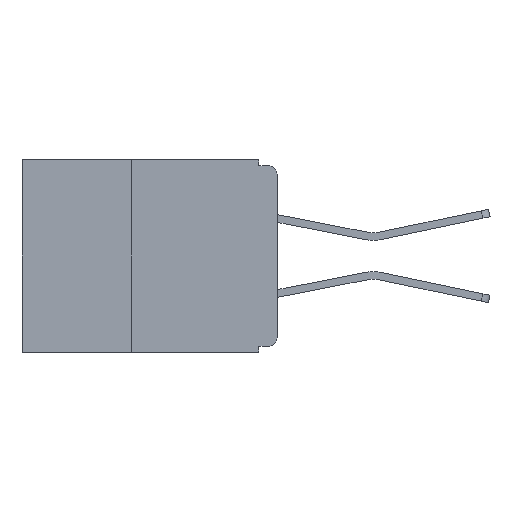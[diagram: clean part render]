
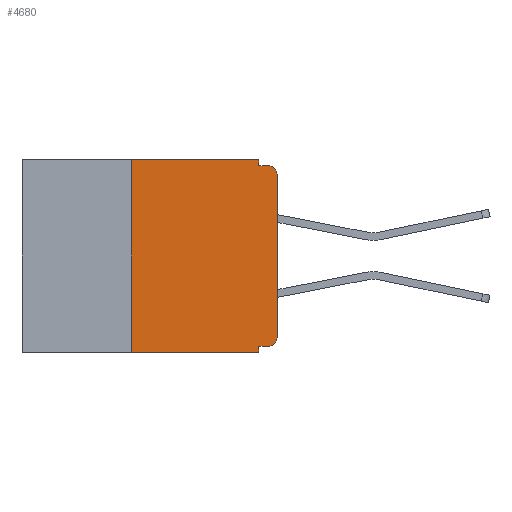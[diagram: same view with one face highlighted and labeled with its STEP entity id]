
A CAD part, left-side view. The second image highlights one B-rep face of the part: STEP entity #4680.
In plain terms, the highlighted planar face has unit normal (-1, 0, 0).
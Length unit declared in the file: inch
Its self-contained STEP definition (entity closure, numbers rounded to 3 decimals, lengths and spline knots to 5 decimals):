
#2693 = LINE ( 'NONE', #8300, #17090 ) ;
#2727 = DIRECTION ( 'NONE',  ( 0., 0., -1. ) ) ;
#2746 = DIRECTION ( 'NONE',  ( 1., 0., 0. ) ) ;
#2768 = CARTESIAN_POINT ( 'NONE',  ( 0., 0.437, 0. ) ) ;
#2789 = DIRECTION ( 'NONE',  ( 0., 0., 1. ) ) ;
#2820 = PLANE ( 'NONE',  #5683 ) ;
#3290 = VERTEX_POINT ( 'NONE', #14722 ) ;
#3549 = LINE ( 'NONE', #13092, #12938 ) ;
#3999 = CARTESIAN_POINT ( 'NONE',  ( 0., 0.031, -0.33 ) ) ;
#4013 = VERTEX_POINT ( 'NONE', #18665 ) ;
#4026 = VERTEX_POINT ( 'NONE', #16457 ) ;
#4680 = ADVANCED_FACE ( 'NONE', ( #7661 ), #2820, .F. ) ;
#4842 = VERTEX_POINT ( 'NONE', #9353 ) ;
#5357 = CARTESIAN_POINT ( 'NONE',  ( 0., 0., -0.32 ) ) ;
#5683 = AXIS2_PLACEMENT_3D ( 'NONE', #2768, #2746, #2727 ) ;
#5891 = DIRECTION ( 'NONE',  ( 0., 0., -1. ) ) ;
#5991 = ORIENTED_EDGE ( 'NONE', *, *, #6027, .T. ) ;
#6027 = EDGE_CURVE ( 'NONE', #11370, #3290, #3549, .T. ) ;
#6290 = VECTOR ( 'NONE', #13671, 39.37008 ) ;
#6608 = ORIENTED_EDGE ( 'NONE', *, *, #19574, .F. ) ;
#6658 = ORIENTED_EDGE ( 'NONE', *, *, #15875, .F. ) ;
#6917 = VECTOR ( 'NONE', #16677, 39.37008 ) ;
#7036 = EDGE_CURVE ( 'NONE', #18478, #4026, #2693, .T. ) ;
#7337 = LINE ( 'NONE', #14040, #17340 ) ;
#7353 = VERTEX_POINT ( 'NONE', #21241 ) ;
#7435 = LINE ( 'NONE', #19151, #6290 ) ;
#7532 = EDGE_CURVE ( 'NONE', #7353, #4013, #7640, .T. ) ;
#7640 = LINE ( 'NONE', #16915, #17066 ) ;
#7661 = FACE_OUTER_BOUND ( 'NONE', #16410, .T. ) ;
#7662 = DIRECTION ( 'NONE',  ( 0., -1., 0. ) ) ;
#7766 = VERTEX_POINT ( 'NONE', #11839 ) ;
#8300 = CARTESIAN_POINT ( 'NONE',  ( 0., 0.437, -0.33 ) ) ;
#8378 = DIRECTION ( 'NONE',  ( 0., -1., 0. ) ) ;
#8676 = CARTESIAN_POINT ( 'NONE',  ( 0., 0.25, -0.33 ) ) ;
#9353 = CARTESIAN_POINT ( 'NONE',  ( 0., 0.25, 0. ) ) ;
#9456 = ORIENTED_EDGE ( 'NONE', *, *, #7036, .T. ) ;
#9535 = ORIENTED_EDGE ( 'NONE', *, *, #11636, .F. ) ;
#9562 = LINE ( 'NONE', #3999, #23712 ) ;
#10077 = CARTESIAN_POINT ( 'NONE',  ( 0., 0.015, -0.305 ) ) ;
#10158 = CARTESIAN_POINT ( 'NONE',  ( 0., 0.015, -0.025 ) ) ;
#10214 = EDGE_CURVE ( 'NONE', #7766, #20772, #12521, .T. ) ;
#11170 = EDGE_CURVE ( 'NONE', #7766, #11370, #12478, .T. ) ;
#11370 = VERTEX_POINT ( 'NONE', #22067 ) ;
#11619 = VECTOR ( 'NONE', #8378, 39.37008 ) ;
#11636 = EDGE_CURVE ( 'NONE', #23895, #7353, #7435, .T. ) ;
#11839 = CARTESIAN_POINT ( 'NONE',  ( 0., 0.015, -0.32 ) ) ;
#11883 = AXIS2_PLACEMENT_3D ( 'NONE', #10158, #23100, #12053 ) ;
#11970 = DIRECTION ( 'NONE',  ( 0., 0., -1. ) ) ;
#12053 = DIRECTION ( 'NONE',  ( 0., 0., -1. ) ) ;
#12228 = ORIENTED_EDGE ( 'NONE', *, *, #18784, .F. ) ;
#12478 = CIRCLE ( 'NONE', #20445, 0.015 ) ;
#12521 = LINE ( 'NONE', #5357, #6917 ) ;
#12926 = DIRECTION ( 'NONE',  ( 0., 0., 1. ) ) ;
#12938 = VECTOR ( 'NONE', #12926, 39.37008 ) ;
#13092 = CARTESIAN_POINT ( 'NONE',  ( 0., 0., 0. ) ) ;
#13671 = DIRECTION ( 'NONE',  ( 0., 0., -1. ) ) ;
#13830 = ORIENTED_EDGE ( 'NONE', *, *, #10214, .F. ) ;
#13922 = ORIENTED_EDGE ( 'NONE', *, *, #7532, .F. ) ;
#13981 = CARTESIAN_POINT ( 'NONE',  ( 0., 0.031, 0. ) ) ;
#14040 = CARTESIAN_POINT ( 'NONE',  ( 0., 0.25, -0.33 ) ) ;
#14476 = ORIENTED_EDGE ( 'NONE', *, *, #11170, .T. ) ;
#14722 = CARTESIAN_POINT ( 'NONE',  ( 0., 0., -0.025 ) ) ;
#15875 = EDGE_CURVE ( 'NONE', #18478, #4842, #7337, .T. ) ;
#16245 = DIRECTION ( 'NONE',  ( 0., -1., 0. ) ) ;
#16410 = EDGE_LOOP ( 'NONE', ( #5991, #22566, #13922, #9535, #6608, #6658, #9456, #12228, #13830, #14476 ) ) ;
#16457 = CARTESIAN_POINT ( 'NONE',  ( 0., 0.031, -0.33 ) ) ;
#16677 = DIRECTION ( 'NONE',  ( 0., 1., 0. ) ) ;
#16765 = CIRCLE ( 'NONE', #11883, 0.015 ) ;
#16915 = CARTESIAN_POINT ( 'NONE',  ( 0., 0., -0.01 ) ) ;
#17066 = VECTOR ( 'NONE', #16245, 39.37008 ) ;
#17090 = VECTOR ( 'NONE', #7662, 39.37008 ) ;
#17340 = VECTOR ( 'NONE', #2789, 39.37008 ) ;
#18478 = VERTEX_POINT ( 'NONE', #8676 ) ;
#18665 = CARTESIAN_POINT ( 'NONE',  ( 0., 0.015, -0.01 ) ) ;
#18784 = EDGE_CURVE ( 'NONE', #20772, #4026, #9562, .T. ) ;
#19151 = CARTESIAN_POINT ( 'NONE',  ( 0., 0.031, 0. ) ) ;
#19521 = CARTESIAN_POINT ( 'NONE',  ( 0., 0.437, 0. ) ) ;
#19574 = EDGE_CURVE ( 'NONE', #4842, #23895, #20294, .T. ) ;
#19692 = CARTESIAN_POINT ( 'NONE',  ( 0., 0.031, -0.32 ) ) ;
#20294 = LINE ( 'NONE', #19521, #11619 ) ;
#20445 = AXIS2_PLACEMENT_3D ( 'NONE', #10077, #23019, #11970 ) ;
#20772 = VERTEX_POINT ( 'NONE', #19692 ) ;
#21241 = CARTESIAN_POINT ( 'NONE',  ( 0., 0.031, -0.01 ) ) ;
#21878 = EDGE_CURVE ( 'NONE', #3290, #4013, #16765, .T. ) ;
#22067 = CARTESIAN_POINT ( 'NONE',  ( 0., 0., -0.305 ) ) ;
#22566 = ORIENTED_EDGE ( 'NONE', *, *, #21878, .T. ) ;
#23019 = DIRECTION ( 'NONE',  ( -1., 0., 0. ) ) ;
#23100 = DIRECTION ( 'NONE',  ( -1., 0., 0. ) ) ;
#23712 = VECTOR ( 'NONE', #5891, 39.37008 ) ;
#23895 = VERTEX_POINT ( 'NONE', #13981 ) ;
